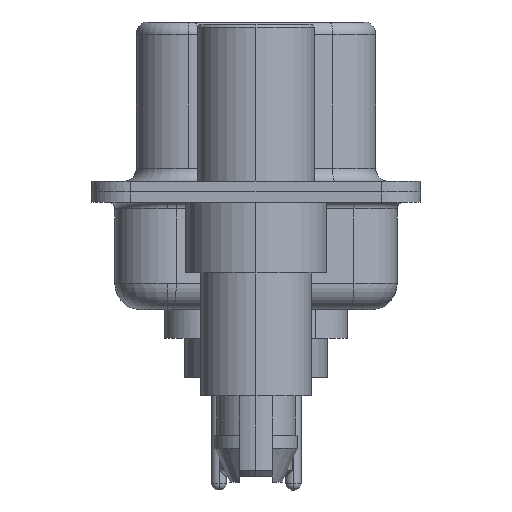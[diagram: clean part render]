
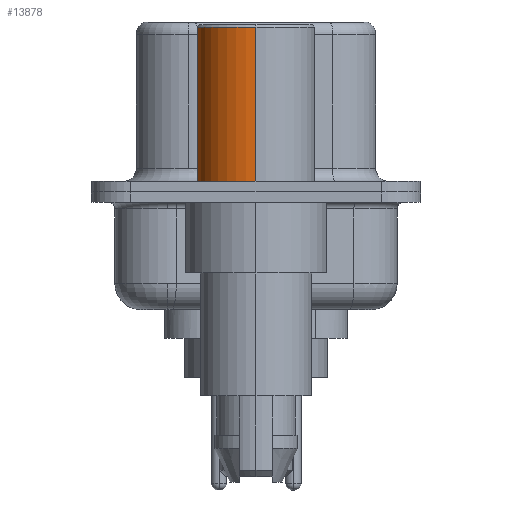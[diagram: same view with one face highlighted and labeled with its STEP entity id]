
A CAD part, left-side view. The second image highlights one B-rep face of the part: STEP entity #13878.
In plain terms, the highlighted cylindrical face has radius 2.25 mm (diameter 4.5 mm), a partial arc.
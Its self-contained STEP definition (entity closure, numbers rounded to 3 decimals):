
#102 = CARTESIAN_POINT ( 'NONE',  ( 0., 0., 0.4 ) ) ;
#312 = CARTESIAN_POINT ( 'NONE',  ( -2.25, 0., 6.3 ) ) ;
#1833 = EDGE_CURVE ( 'NONE', #3068, #12379, #6403, .T. ) ;
#1901 = DIRECTION ( 'NONE',  ( 0., 0., 1. ) ) ;
#1936 = CARTESIAN_POINT ( 'NONE',  ( 2.25, 0., 0.581 ) ) ;
#2141 = EDGE_CURVE ( 'NONE', #3050, #20398, #13307, .T. ) ;
#2216 = AXIS2_PLACEMENT_3D ( 'NONE', #6664, #11995, #13789 ) ;
#2385 = VECTOR ( 'NONE', #16205, 1000. ) ;
#3050 = VERTEX_POINT ( 'NONE', #16528 ) ;
#3068 = VERTEX_POINT ( 'NONE', #19565 ) ;
#3223 = LINE ( 'NONE', #1936, #2385 ) ;
#3526 = ORIENTED_EDGE ( 'NONE', *, *, #6702, .F. ) ;
#3700 = VECTOR ( 'NONE', #4906, 1000. ) ;
#3765 = FACE_OUTER_BOUND ( 'NONE', #4441, .T. ) ;
#4414 = ORIENTED_EDGE ( 'NONE', *, *, #8966, .T. ) ;
#4441 = EDGE_LOOP ( 'NONE', ( #12940, #4414, #12199, #3526 ) ) ;
#4906 = DIRECTION ( 'NONE',  ( 0., 0., 1. ) ) ;
#6403 = CIRCLE ( 'NONE', #8404, 2.25 ) ;
#6664 = CARTESIAN_POINT ( 'NONE',  ( 0., 0., 0.581 ) ) ;
#6702 = EDGE_CURVE ( 'NONE', #3050, #3068, #3223, .T. ) ;
#8317 = CARTESIAN_POINT ( 'NONE',  ( -2.25, 0., 0.4 ) ) ;
#8404 = AXIS2_PLACEMENT_3D ( 'NONE', #12482, #1901, #14445 ) ;
#8966 = EDGE_CURVE ( 'NONE', #20398, #12379, #14237, .T. ) ;
#10355 = CARTESIAN_POINT ( 'NONE',  ( -2.25, 0., 0.581 ) ) ;
#11995 = DIRECTION ( 'NONE',  ( 0., 0., 1. ) ) ;
#12199 = ORIENTED_EDGE ( 'NONE', *, *, #1833, .F. ) ;
#12379 = VERTEX_POINT ( 'NONE', #312 ) ;
#12482 = CARTESIAN_POINT ( 'NONE',  ( 0., 0., 6.3 ) ) ;
#12648 = DIRECTION ( 'NONE',  ( 1., 0., 0. ) ) ;
#12940 = ORIENTED_EDGE ( 'NONE', *, *, #2141, .T. ) ;
#13307 = CIRCLE ( 'NONE', #15587, 2.25 ) ;
#13789 = DIRECTION ( 'NONE',  ( 1., 0., 0. ) ) ;
#13878 = ADVANCED_FACE ( 'NONE', ( #3765 ), #17938, .T. ) ;
#14237 = LINE ( 'NONE', #10355, #3700 ) ;
#14445 = DIRECTION ( 'NONE',  ( 1., 0., 0. ) ) ;
#15587 = AXIS2_PLACEMENT_3D ( 'NONE', #102, #16031, #12648 ) ;
#16031 = DIRECTION ( 'NONE',  ( 0., 0., 1. ) ) ;
#16205 = DIRECTION ( 'NONE',  ( 0., 0., 1. ) ) ;
#16528 = CARTESIAN_POINT ( 'NONE',  ( 2.25, 0., 0.4 ) ) ;
#17938 = CYLINDRICAL_SURFACE ( 'NONE', #2216, 2.25 ) ;
#19565 = CARTESIAN_POINT ( 'NONE',  ( 2.25, 0., 6.3 ) ) ;
#20398 = VERTEX_POINT ( 'NONE', #8317 ) ;
